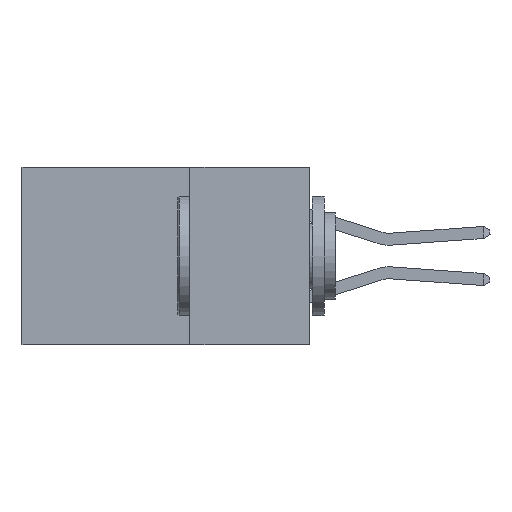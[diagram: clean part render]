
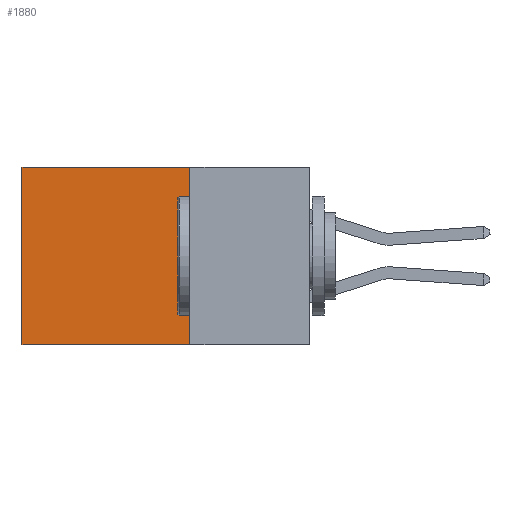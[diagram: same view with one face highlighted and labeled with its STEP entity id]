
A CAD part, left-side view. The second image highlights one B-rep face of the part: STEP entity #1880.
In plain terms, the highlighted planar face has unit normal (-1, 0, 0).
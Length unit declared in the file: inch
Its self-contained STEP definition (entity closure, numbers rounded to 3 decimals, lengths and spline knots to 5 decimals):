
#360 = ORIENTED_EDGE ( 'NONE', *, *, #8029, .T. ) ;
#894 = AXIS2_PLACEMENT_3D ( 'NONE', #5109, #5796, #3703 ) ;
#1014 = DIRECTION ( 'NONE',  ( 0., 1., 0. ) ) ;
#1414 = CARTESIAN_POINT ( 'NONE',  ( 0.2615, 0.25, -0.37 ) ) ;
#1521 = VERTEX_POINT ( 'NONE', #10799 ) ;
#1669 = CARTESIAN_POINT ( 'NONE',  ( 0.2615, 0.6, -0.37 ) ) ;
#1830 = VECTOR ( 'NONE', #1014, 39.37008 ) ;
#1848 = DIRECTION ( 'NONE',  ( 0., 0., -1. ) ) ;
#1880 = ADVANCED_FACE ( 'NONE', ( #10214 ), #6799, .F. ) ;
#2812 = CARTESIAN_POINT ( 'NONE',  ( 0.2615, 0.6, -0.37 ) ) ;
#3010 = EDGE_CURVE ( 'NONE', #4633, #3891, #6979, .T. ) ;
#3703 = DIRECTION ( 'NONE',  ( 0., 0., -1. ) ) ;
#3891 = VERTEX_POINT ( 'NONE', #2812 ) ;
#3912 = CARTESIAN_POINT ( 'NONE',  ( 0.2615, 0.25, 0. ) ) ;
#3954 = DIRECTION ( 'NONE',  ( 0., 1., 0. ) ) ;
#4633 = VERTEX_POINT ( 'NONE', #4662 ) ;
#4662 = CARTESIAN_POINT ( 'NONE',  ( 0.2615, 0.25, -0.37 ) ) ;
#4757 = VECTOR ( 'NONE', #7801, 39.37008 ) ;
#5109 = CARTESIAN_POINT ( 'NONE',  ( 0.2615, 0.25, -0.37 ) ) ;
#5191 = EDGE_LOOP ( 'NONE', ( #360, #9209, #8782, #5529 ) ) ;
#5529 = ORIENTED_EDGE ( 'NONE', *, *, #6306, .T. ) ;
#5689 = LINE ( 'NONE', #1669, #8063 ) ;
#5796 = DIRECTION ( 'NONE',  ( 1., 0., 0. ) ) ;
#6306 = EDGE_CURVE ( 'NONE', #7498, #1521, #10819, .T. ) ;
#6799 = PLANE ( 'NONE',  #894 ) ;
#6979 = LINE ( 'NONE', #1414, #1830 ) ;
#7146 = LINE ( 'NONE', #7325, #4757 ) ;
#7325 = CARTESIAN_POINT ( 'NONE',  ( 0.2615, 0.25, -0.37 ) ) ;
#7498 = VERTEX_POINT ( 'NONE', #10352 ) ;
#7653 = EDGE_CURVE ( 'NONE', #7498, #4633, #7146, .T. ) ;
#7801 = DIRECTION ( 'NONE',  ( 0., 0., -1. ) ) ;
#8029 = EDGE_CURVE ( 'NONE', #1521, #3891, #5689, .T. ) ;
#8063 = VECTOR ( 'NONE', #1848, 39.37008 ) ;
#8565 = VECTOR ( 'NONE', #3954, 39.37008 ) ;
#8782 = ORIENTED_EDGE ( 'NONE', *, *, #7653, .F. ) ;
#9209 = ORIENTED_EDGE ( 'NONE', *, *, #3010, .F. ) ;
#10214 = FACE_OUTER_BOUND ( 'NONE', #5191, .T. ) ;
#10352 = CARTESIAN_POINT ( 'NONE',  ( 0.2615, 0.25, 0. ) ) ;
#10799 = CARTESIAN_POINT ( 'NONE',  ( 0.2615, 0.6, 0. ) ) ;
#10819 = LINE ( 'NONE', #3912, #8565 ) ;
